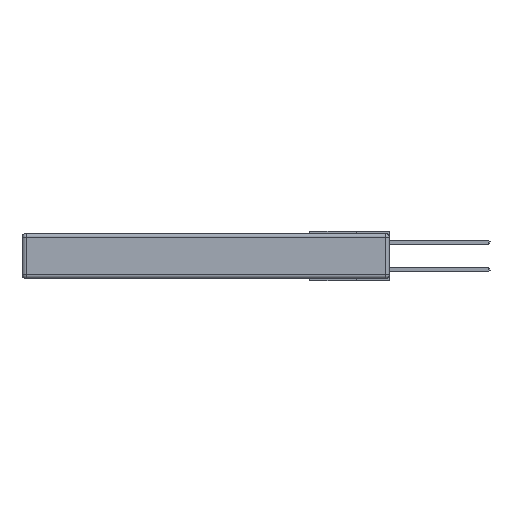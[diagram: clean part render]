
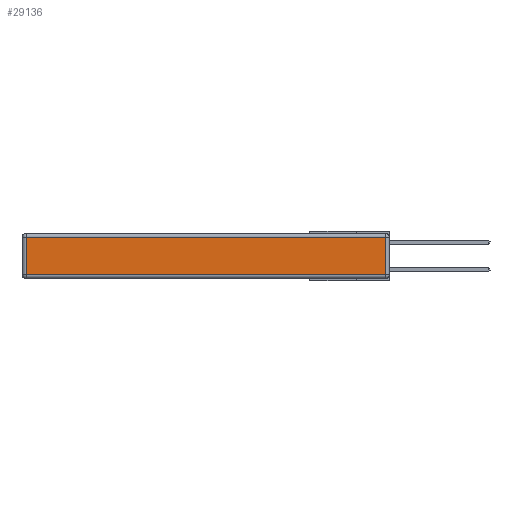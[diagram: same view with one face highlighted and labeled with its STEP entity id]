
A CAD part, left-side view. The second image highlights one B-rep face of the part: STEP entity #29136.
In plain terms, the highlighted planar face has unit normal (-1, 0, 0).
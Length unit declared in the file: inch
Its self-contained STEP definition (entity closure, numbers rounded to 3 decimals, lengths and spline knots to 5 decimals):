
#1759 = ORIENTED_EDGE ( 'NONE', *, *, #31519, .T. ) ;
#2281 = EDGE_CURVE ( 'NONE', #25511, #25112, #5935, .T. ) ;
#4622 = VERTEX_POINT ( 'NONE', #31990 ) ;
#5885 = DIRECTION ( 'NONE',  ( -1., 0., 0. ) ) ;
#5935 = LINE ( 'NONE', #33049, #15920 ) ;
#8712 = EDGE_CURVE ( 'NONE', #4622, #11377, #30487, .T. ) ;
#11377 = VERTEX_POINT ( 'NONE', #25988 ) ;
#13028 = EDGE_CURVE ( 'NONE', #11377, #25511, #31023, .T. ) ;
#13911 = DIRECTION ( 'NONE',  ( 0., 0., -1. ) ) ;
#14320 = VECTOR ( 'NONE', #30102, 39.37008 ) ;
#15616 = CARTESIAN_POINT ( 'NONE',  ( 0., 0.03, -0.343 ) ) ;
#15920 = VECTOR ( 'NONE', #13911, 39.37008 ) ;
#16155 = ORIENTED_EDGE ( 'NONE', *, *, #2281, .T. ) ;
#19251 = CARTESIAN_POINT ( 'NONE',  ( 0., 0., -0.343 ) ) ;
#19702 = ORIENTED_EDGE ( 'NONE', *, *, #13028, .T. ) ;
#20825 = AXIS2_PLACEMENT_3D ( 'NONE', #19251, #5885, #24539 ) ;
#24539 = DIRECTION ( 'NONE',  ( 0., 0., 1. ) ) ;
#24872 = CARTESIAN_POINT ( 'NONE',  ( 0., 2.72, -0.03 ) ) ;
#24987 = CARTESIAN_POINT ( 'NONE',  ( 0., 2.75, -0.03 ) ) ;
#25112 = VERTEX_POINT ( 'NONE', #26310 ) ;
#25485 = VECTOR ( 'NONE', #28591, 39.37008 ) ;
#25511 = VERTEX_POINT ( 'NONE', #24872 ) ;
#25988 = CARTESIAN_POINT ( 'NONE',  ( 0., 0.03, -0.03 ) ) ;
#26310 = CARTESIAN_POINT ( 'NONE',  ( 0., 2.72, -0.313 ) ) ;
#26829 = CARTESIAN_POINT ( 'NONE',  ( 0., 0., -0.313 ) ) ;
#26941 = DIRECTION ( 'NONE',  ( 0., -1., 0. ) ) ;
#28591 = DIRECTION ( 'NONE',  ( 0., 0., 1. ) ) ;
#29136 = ADVANCED_FACE ( 'NONE', ( #31065 ), #29748, .T. ) ;
#29748 = PLANE ( 'NONE',  #20825 ) ;
#30102 = DIRECTION ( 'NONE',  ( 0., 1., 0. ) ) ;
#30487 = LINE ( 'NONE', #15616, #25485 ) ;
#31023 = LINE ( 'NONE', #24987, #14320 ) ;
#31065 = FACE_OUTER_BOUND ( 'NONE', #31478, .T. ) ;
#31478 = EDGE_LOOP ( 'NONE', ( #1759, #32057, #19702, #16155 ) ) ;
#31519 = EDGE_CURVE ( 'NONE', #25112, #4622, #34322, .T. ) ;
#31813 = VECTOR ( 'NONE', #26941, 39.37008 ) ;
#31990 = CARTESIAN_POINT ( 'NONE',  ( 0., 0.03, -0.313 ) ) ;
#32057 = ORIENTED_EDGE ( 'NONE', *, *, #8712, .T. ) ;
#33049 = CARTESIAN_POINT ( 'NONE',  ( 0., 2.72, -0.343 ) ) ;
#34322 = LINE ( 'NONE', #26829, #31813 ) ;
